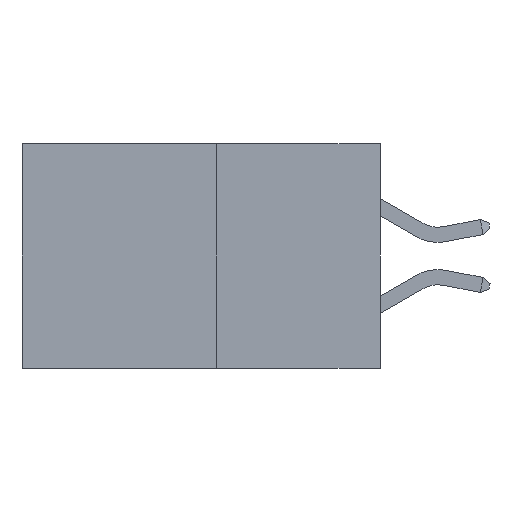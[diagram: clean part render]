
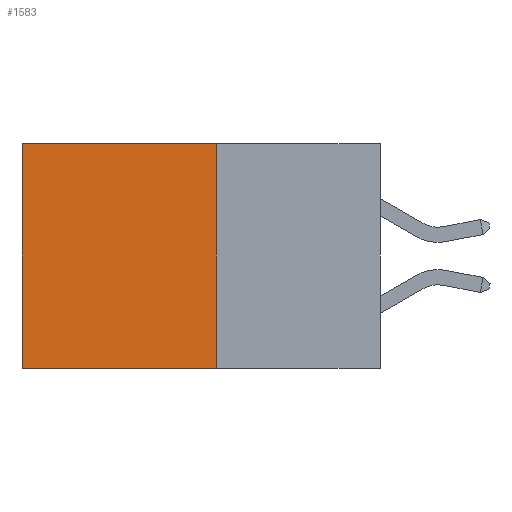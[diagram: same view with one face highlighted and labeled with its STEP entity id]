
A CAD part, left-side view. The second image highlights one B-rep face of the part: STEP entity #1583.
In plain terms, the highlighted planar face has unit normal (-1, 0, 0).
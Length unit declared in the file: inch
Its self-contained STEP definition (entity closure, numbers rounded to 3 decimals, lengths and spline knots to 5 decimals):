
#134 = EDGE_LOOP ( 'NONE', ( #1444, #12593, #7642, #3386 ) ) ;
#286 = LINE ( 'NONE', #4652, #9624 ) ;
#652 = LINE ( 'NONE', #10273, #4012 ) ;
#769 = VERTEX_POINT ( 'NONE', #14010 ) ;
#1153 = VERTEX_POINT ( 'NONE', #14684 ) ;
#1444 = ORIENTED_EDGE ( 'NONE', *, *, #2077, .T. ) ;
#1583 = ADVANCED_FACE ( 'NONE', ( #6705 ), #6438, .F. ) ;
#1941 = LINE ( 'NONE', #3598, #14136 ) ;
#2077 = EDGE_CURVE ( 'NONE', #4161, #1153, #286, .T. ) ;
#3386 = ORIENTED_EDGE ( 'NONE', *, *, #9778, .T. ) ;
#3558 = EDGE_CURVE ( 'NONE', #9721, #1153, #1941, .T. ) ;
#3598 = CARTESIAN_POINT ( 'NONE',  ( 0.277, 0.27, -0.37 ) ) ;
#4012 = VECTOR ( 'NONE', #9124, 39.37008 ) ;
#4161 = VERTEX_POINT ( 'NONE', #10568 ) ;
#4652 = CARTESIAN_POINT ( 'NONE',  ( 0.277, 0.59, -0.37 ) ) ;
#6350 = DIRECTION ( 'NONE',  ( 0., 0., -1. ) ) ;
#6379 = DIRECTION ( 'NONE',  ( 1., 0., 0. ) ) ;
#6438 = PLANE ( 'NONE',  #13620 ) ;
#6542 = CARTESIAN_POINT ( 'NONE',  ( 0.277, 0.27, -0.37 ) ) ;
#6705 = FACE_OUTER_BOUND ( 'NONE', #134, .T. ) ;
#6947 = DIRECTION ( 'NONE',  ( 0., 0., -1. ) ) ;
#7400 = EDGE_CURVE ( 'NONE', #769, #9721, #13070, .T. ) ;
#7632 = VECTOR ( 'NONE', #6947, 39.37008 ) ;
#7642 = ORIENTED_EDGE ( 'NONE', *, *, #7400, .F. ) ;
#9076 = CARTESIAN_POINT ( 'NONE',  ( 0.277, 0.27, -0.37 ) ) ;
#9124 = DIRECTION ( 'NONE',  ( 0., 1., 0. ) ) ;
#9415 = DIRECTION ( 'NONE',  ( 0., 0., -1. ) ) ;
#9624 = VECTOR ( 'NONE', #9415, 39.37008 ) ;
#9721 = VERTEX_POINT ( 'NONE', #9076 ) ;
#9778 = EDGE_CURVE ( 'NONE', #769, #4161, #652, .T. ) ;
#10273 = CARTESIAN_POINT ( 'NONE',  ( 0.277, 0.27, 0. ) ) ;
#10568 = CARTESIAN_POINT ( 'NONE',  ( 0.277, 0.59, 0. ) ) ;
#12593 = ORIENTED_EDGE ( 'NONE', *, *, #3558, .F. ) ;
#12749 = CARTESIAN_POINT ( 'NONE',  ( 0.277, 0.27, -0.37 ) ) ;
#13070 = LINE ( 'NONE', #12749, #7632 ) ;
#13620 = AXIS2_PLACEMENT_3D ( 'NONE', #6542, #6379, #6350 ) ;
#14010 = CARTESIAN_POINT ( 'NONE',  ( 0.277, 0.27, 0. ) ) ;
#14136 = VECTOR ( 'NONE', #14248, 39.37008 ) ;
#14248 = DIRECTION ( 'NONE',  ( 0., 1., 0. ) ) ;
#14684 = CARTESIAN_POINT ( 'NONE',  ( 0.277, 0.59, -0.37 ) ) ;
